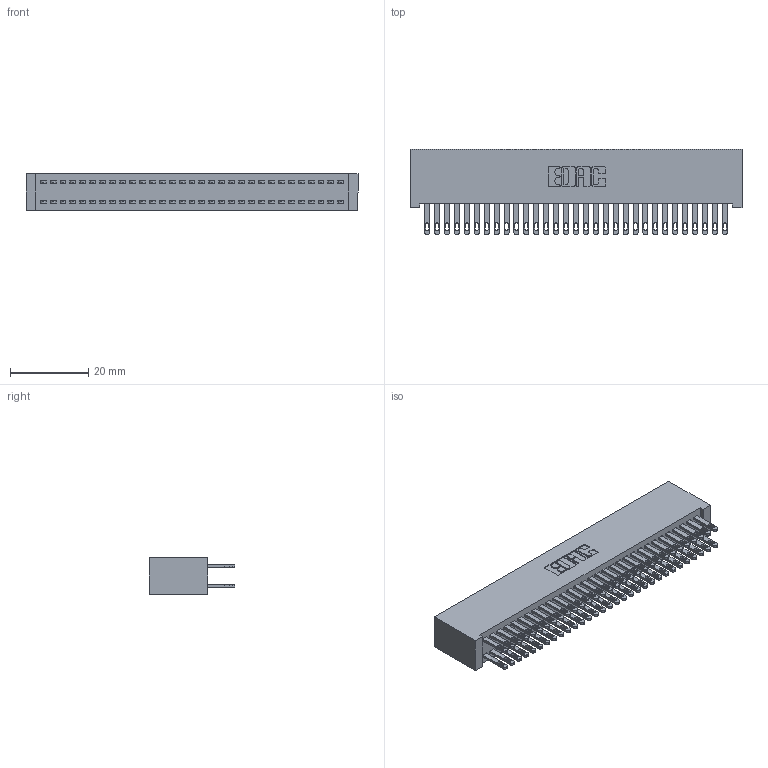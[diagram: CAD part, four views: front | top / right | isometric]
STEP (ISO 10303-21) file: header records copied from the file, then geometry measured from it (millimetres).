
FILE_DESCRIPTION (( 'STEP AP203' ), '1' );
FILE_NAME ('342-062-500-201.STEP', '2018-08-13T06:29:07', ( '' ), ( '' ), 'SwSTEP 2.0', 'SolidWorks 2016', '' );
FILE_SCHEMA (( 'CONFIG_CONTROL_DESIGN' ));
Length unit declared in the file: inch
Products named in the file (3): 342 Part_Lugless; 345-292-001_345-293-100; 342-062-500-201
Assembly tree (63 placements, depth 2):
  342-062-500-201
    342 Part_Lugless
    345-292-001_345-293-100  x62
Bounding box: 84.99 x 21.85 x 9.4 mm (x, y, z)
Volume: 8213.1 mm3; surface area: 14137.7 mm2
Topology: 63 solids, 63 shells, 3078 faces, 9389 edges, 6258 vertices
Faces by surface type: plane 1922, cylinder 1156
Entity records: 20887 total; most frequent: CARTESIAN_POINT 3470, ORIENTED_EDGE 3406, DIRECTION 2979, EDGE_CURVE 1703, LINE 1579, VECTOR 1579, VERTEX_POINT 1134, AXIS2_PLACEMENT_3D 700
